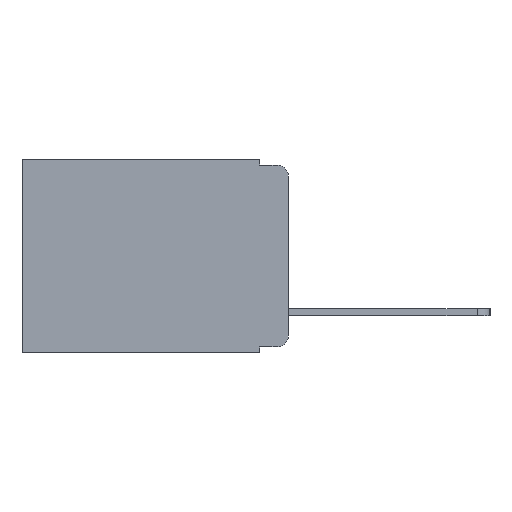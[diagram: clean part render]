
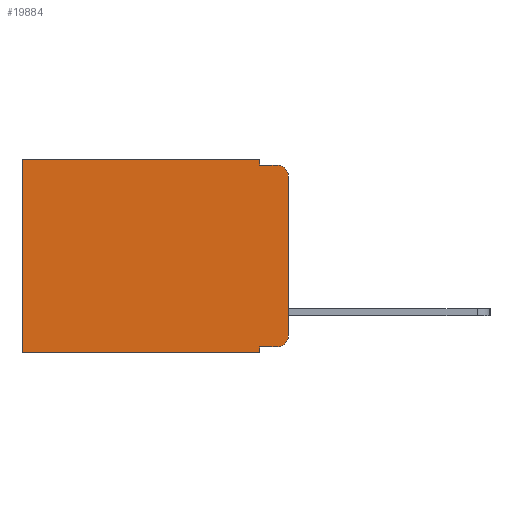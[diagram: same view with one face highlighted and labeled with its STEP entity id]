
A CAD part, left-side view. The second image highlights one B-rep face of the part: STEP entity #19884.
In plain terms, the highlighted planar face has unit normal (-1, 0, 0).
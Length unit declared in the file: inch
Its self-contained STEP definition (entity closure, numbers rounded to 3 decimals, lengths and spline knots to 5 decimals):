
#461 = DIRECTION ( 'NONE',  ( -1., 0., 0. ) ) ;
#646 = VERTEX_POINT ( 'NONE', #11974 ) ;
#869 = VERTEX_POINT ( 'NONE', #21563 ) ;
#1472 = CARTESIAN_POINT ( 'NONE',  ( 0.298, 0.051, 0. ) ) ;
#1573 = EDGE_CURVE ( 'NONE', #646, #4521, #8005, .T. ) ;
#2141 = CARTESIAN_POINT ( 'NONE',  ( 0.298, 0.02, -0.333 ) ) ;
#2187 = VERTEX_POINT ( 'NONE', #2141 ) ;
#2585 = CARTESIAN_POINT ( 'NONE',  ( 0.298, 0.051, -0.333 ) ) ;
#2724 = EDGE_CURVE ( 'NONE', #7439, #19154, #20681, .T. ) ;
#2752 = VECTOR ( 'NONE', #9379, 39.37008 ) ;
#3004 = CARTESIAN_POINT ( 'NONE',  ( 0.298, 0., 0. ) ) ;
#3325 = LINE ( 'NONE', #16480, #2752 ) ;
#3365 = CARTESIAN_POINT ( 'NONE',  ( 0.298, 0.473, 0. ) ) ;
#3682 = LINE ( 'NONE', #10925, #12570 ) ;
#4383 = CARTESIAN_POINT ( 'NONE',  ( 0.298, 0.02, -0.03 ) ) ;
#4520 = EDGE_CURVE ( 'NONE', #12424, #15335, #3682, .T. ) ;
#4521 = VERTEX_POINT ( 'NONE', #21532 ) ;
#4579 = ORIENTED_EDGE ( 'NONE', *, *, #20076, .F. ) ;
#4836 = CARTESIAN_POINT ( 'NONE',  ( 0.298, 0.051, -0.01 ) ) ;
#5197 = AXIS2_PLACEMENT_3D ( 'NONE', #11129, #461, #12915 ) ;
#5281 = CARTESIAN_POINT ( 'NONE',  ( 0.298, 0.473, -0.343 ) ) ;
#6223 = DIRECTION ( 'NONE',  ( 0., 0., -1. ) ) ;
#6259 = VERTEX_POINT ( 'NONE', #4836 ) ;
#6583 = VECTOR ( 'NONE', #16310, 39.37008 ) ;
#6667 = DIRECTION ( 'NONE',  ( 0., 1., 0. ) ) ;
#6916 = EDGE_CURVE ( 'NONE', #12424, #2187, #22963, .T. ) ;
#7176 = CARTESIAN_POINT ( 'NONE',  ( 0.298, 0., 0. ) ) ;
#7225 = CIRCLE ( 'NONE', #5197, 0.02 ) ;
#7356 = ORIENTED_EDGE ( 'NONE', *, *, #6916, .T. ) ;
#7439 = VERTEX_POINT ( 'NONE', #3365 ) ;
#7630 = ORIENTED_EDGE ( 'NONE', *, *, #1573, .F. ) ;
#8005 = LINE ( 'NONE', #22627, #21543 ) ;
#8404 = DIRECTION ( 'NONE',  ( 0., -1., 0. ) ) ;
#8462 = CIRCLE ( 'NONE', #11022, 0.02 ) ;
#8475 = VECTOR ( 'NONE', #8404, 39.37008 ) ;
#8934 = DIRECTION ( 'NONE',  ( 1., 0., 0. ) ) ;
#9021 = LINE ( 'NONE', #22542, #8475 ) ;
#9379 = DIRECTION ( 'NONE',  ( 0., 0., -1. ) ) ;
#9829 = ORIENTED_EDGE ( 'NONE', *, *, #11121, .T. ) ;
#10243 = VECTOR ( 'NONE', #6667, 39.37008 ) ;
#10925 = CARTESIAN_POINT ( 'NONE',  ( 0.298, 0.051, 0. ) ) ;
#10940 = ORIENTED_EDGE ( 'NONE', *, *, #16272, .F. ) ;
#11006 = DIRECTION ( 'NONE',  ( 0., 0., -1. ) ) ;
#11022 = AXIS2_PLACEMENT_3D ( 'NONE', #4383, #16740, #6223 ) ;
#11121 = EDGE_CURVE ( 'NONE', #14487, #7439, #19083, .T. ) ;
#11129 = CARTESIAN_POINT ( 'NONE',  ( 0.298, 0.02, -0.313 ) ) ;
#11404 = FACE_OUTER_BOUND ( 'NONE', #13879, .T. ) ;
#11498 = ORIENTED_EDGE ( 'NONE', *, *, #4520, .F. ) ;
#11546 = DIRECTION ( 'NONE',  ( 0., -1., 0. ) ) ;
#11820 = DIRECTION ( 'NONE',  ( 0., 0., -1. ) ) ;
#11974 = CARTESIAN_POINT ( 'NONE',  ( 0.298, 0., -0.03 ) ) ;
#12424 = VERTEX_POINT ( 'NONE', #21278 ) ;
#12493 = VECTOR ( 'NONE', #13027, 39.37008 ) ;
#12570 = VECTOR ( 'NONE', #11006, 39.37008 ) ;
#12915 = DIRECTION ( 'NONE',  ( 0., 0., -1. ) ) ;
#13027 = DIRECTION ( 'NONE',  ( 0., 1., 0. ) ) ;
#13879 = EDGE_LOOP ( 'NONE', ( #7630, #21734, #18118, #4579, #9829, #15098, #10940, #11498, #7356, #16735 ) ) ;
#14487 = VERTEX_POINT ( 'NONE', #1472 ) ;
#14583 = CARTESIAN_POINT ( 'NONE',  ( 0.298, 0.051, -0.343 ) ) ;
#15098 = ORIENTED_EDGE ( 'NONE', *, *, #2724, .T. ) ;
#15335 = VERTEX_POINT ( 'NONE', #14583 ) ;
#16272 = EDGE_CURVE ( 'NONE', #15335, #19154, #21912, .T. ) ;
#16310 = DIRECTION ( 'NONE',  ( 0., 0., -1. ) ) ;
#16480 = CARTESIAN_POINT ( 'NONE',  ( 0.298, 0.051, 0. ) ) ;
#16540 = CARTESIAN_POINT ( 'NONE',  ( 0.298, 0., -0.343 ) ) ;
#16590 = VECTOR ( 'NONE', #11546, 39.37008 ) ;
#16735 = ORIENTED_EDGE ( 'NONE', *, *, #20797, .T. ) ;
#16740 = DIRECTION ( 'NONE',  ( -1., 0., 0. ) ) ;
#17668 = EDGE_CURVE ( 'NONE', #6259, #869, #9021, .T. ) ;
#17723 = PLANE ( 'NONE',  #19968 ) ;
#18022 = CARTESIAN_POINT ( 'NONE',  ( 0.298, 0.473, 0. ) ) ;
#18118 = ORIENTED_EDGE ( 'NONE', *, *, #17668, .F. ) ;
#19083 = LINE ( 'NONE', #3004, #10243 ) ;
#19154 = VERTEX_POINT ( 'NONE', #5281 ) ;
#19884 = ADVANCED_FACE ( 'NONE', ( #11404 ), #17723, .F. ) ;
#19968 = AXIS2_PLACEMENT_3D ( 'NONE', #7176, #8934, #21320 ) ;
#20076 = EDGE_CURVE ( 'NONE', #14487, #6259, #3325, .T. ) ;
#20681 = LINE ( 'NONE', #18022, #6583 ) ;
#20797 = EDGE_CURVE ( 'NONE', #2187, #4521, #7225, .T. ) ;
#21278 = CARTESIAN_POINT ( 'NONE',  ( 0.298, 0.051, -0.333 ) ) ;
#21320 = DIRECTION ( 'NONE',  ( 0., 0., -1. ) ) ;
#21532 = CARTESIAN_POINT ( 'NONE',  ( 0.298, 0., -0.313 ) ) ;
#21543 = VECTOR ( 'NONE', #11820, 39.37008 ) ;
#21563 = CARTESIAN_POINT ( 'NONE',  ( 0.298, 0.02, -0.01 ) ) ;
#21734 = ORIENTED_EDGE ( 'NONE', *, *, #22434, .T. ) ;
#21912 = LINE ( 'NONE', #16540, #12493 ) ;
#22434 = EDGE_CURVE ( 'NONE', #646, #869, #8462, .T. ) ;
#22542 = CARTESIAN_POINT ( 'NONE',  ( 0.298, 0.051, -0.01 ) ) ;
#22627 = CARTESIAN_POINT ( 'NONE',  ( 0.298, 0., 0. ) ) ;
#22963 = LINE ( 'NONE', #2585, #16590 ) ;
